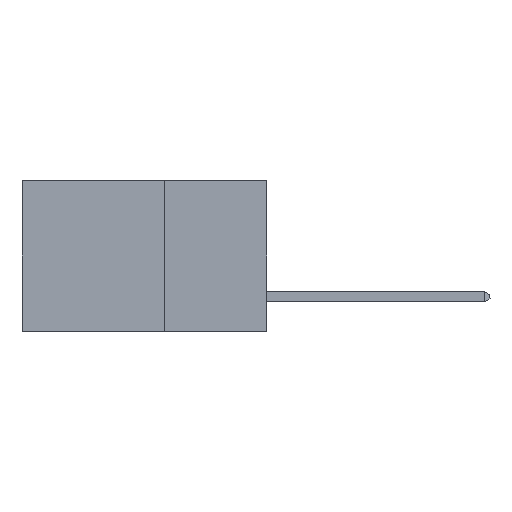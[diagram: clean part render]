
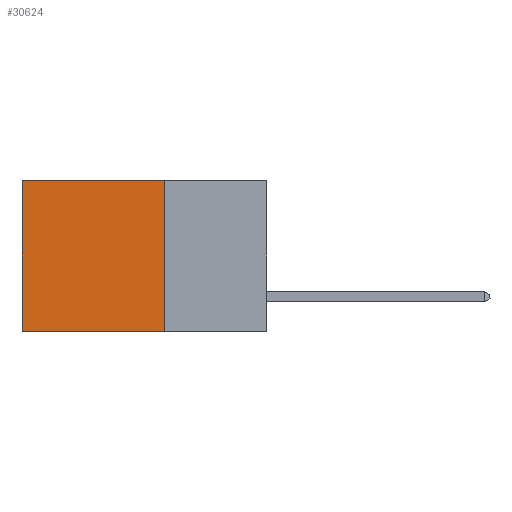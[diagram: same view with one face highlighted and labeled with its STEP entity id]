
A CAD part, left-side view. The second image highlights one B-rep face of the part: STEP entity #30624.
In plain terms, the highlighted planar face has unit normal (-1, 0, 0).
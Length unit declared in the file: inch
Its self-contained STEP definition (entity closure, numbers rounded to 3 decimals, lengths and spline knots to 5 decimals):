
#854 = VECTOR ( 'NONE', #4850, 39.37008 ) ;
#2241 = CARTESIAN_POINT ( 'NONE',  ( 0.2875, 0.25, -0.37 ) ) ;
#3604 = VERTEX_POINT ( 'NONE', #24804 ) ;
#4765 = DIRECTION ( 'NONE',  ( 0., 1., 0. ) ) ;
#4850 = DIRECTION ( 'NONE',  ( 0., 1., 0. ) ) ;
#5031 = DIRECTION ( 'NONE',  ( 0., 0., -1. ) ) ;
#6715 = CARTESIAN_POINT ( 'NONE',  ( 0.2875, 0.25, 0. ) ) ;
#6775 = CARTESIAN_POINT ( 'NONE',  ( 0.2875, 0.25, 0. ) ) ;
#6946 = CARTESIAN_POINT ( 'NONE',  ( 0.2875, 0.25, 0. ) ) ;
#7205 = VECTOR ( 'NONE', #5031, 39.37008 ) ;
#7461 = LINE ( 'NONE', #14458, #854 ) ;
#7516 = EDGE_CURVE ( 'NONE', #8687, #19539, #21457, .T. ) ;
#8687 = VERTEX_POINT ( 'NONE', #6715 ) ;
#8791 = VECTOR ( 'NONE', #21083, 39.37008 ) ;
#9218 = CARTESIAN_POINT ( 'NONE',  ( 0.2875, 0.6, -0.37 ) ) ;
#9402 = DIRECTION ( 'NONE',  ( 0., 0., -1. ) ) ;
#11830 = CARTESIAN_POINT ( 'NONE',  ( 0.2875, 0.25, -0.37 ) ) ;
#12221 = AXIS2_PLACEMENT_3D ( 'NONE', #6946, #23641, #9402 ) ;
#14317 = ORIENTED_EDGE ( 'NONE', *, *, #16779, .T. ) ;
#14458 = CARTESIAN_POINT ( 'NONE',  ( 0.2875, 0.25, 0. ) ) ;
#16779 = EDGE_CURVE ( 'NONE', #3604, #28853, #26205, .T. ) ;
#18919 = EDGE_CURVE ( 'NONE', #8687, #3604, #7461, .T. ) ;
#19426 = CARTESIAN_POINT ( 'NONE',  ( 0.2875, 0.6, 0. ) ) ;
#19539 = VERTEX_POINT ( 'NONE', #11830 ) ;
#21083 = DIRECTION ( 'NONE',  ( 0., 0., -1. ) ) ;
#21246 = PLANE ( 'NONE',  #12221 ) ;
#21457 = LINE ( 'NONE', #6775, #8791 ) ;
#22115 = FACE_OUTER_BOUND ( 'NONE', #25517, .T. ) ;
#22924 = EDGE_CURVE ( 'NONE', #19539, #28853, #25476, .T. ) ;
#23641 = DIRECTION ( 'NONE',  ( 1., 0., 0. ) ) ;
#24743 = VECTOR ( 'NONE', #4765, 39.37008 ) ;
#24804 = CARTESIAN_POINT ( 'NONE',  ( 0.2875, 0.6, 0. ) ) ;
#25476 = LINE ( 'NONE', #2241, #24743 ) ;
#25517 = EDGE_LOOP ( 'NONE', ( #14317, #30317, #28953, #29264 ) ) ;
#26205 = LINE ( 'NONE', #19426, #7205 ) ;
#28853 = VERTEX_POINT ( 'NONE', #9218 ) ;
#28953 = ORIENTED_EDGE ( 'NONE', *, *, #7516, .F. ) ;
#29264 = ORIENTED_EDGE ( 'NONE', *, *, #18919, .T. ) ;
#30317 = ORIENTED_EDGE ( 'NONE', *, *, #22924, .F. ) ;
#30624 = ADVANCED_FACE ( 'NONE', ( #22115 ), #21246, .F. ) ;
